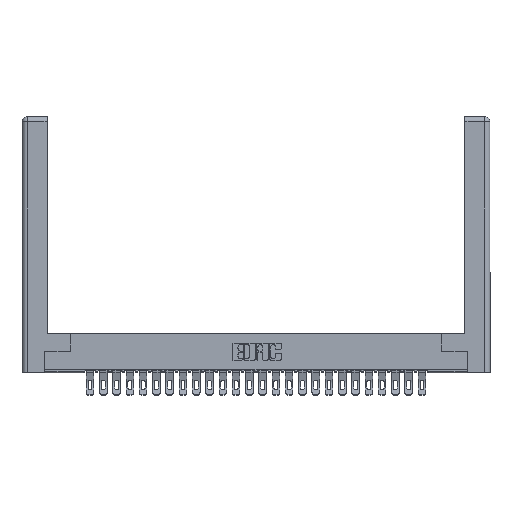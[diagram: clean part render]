
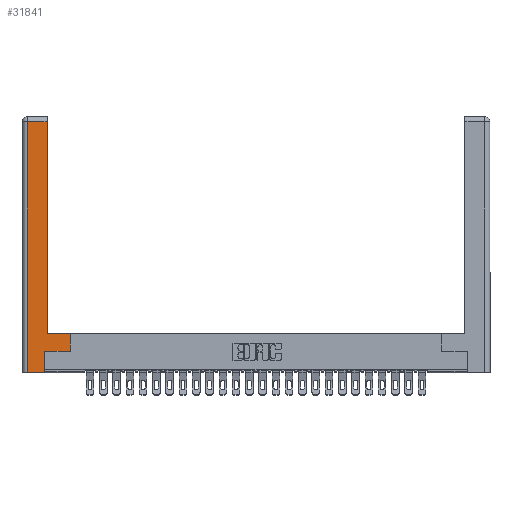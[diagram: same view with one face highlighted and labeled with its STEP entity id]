
A CAD part, top view. The second image highlights one B-rep face of the part: STEP entity #31841.
In plain terms, the highlighted planar face has unit normal (0, 0, 1).
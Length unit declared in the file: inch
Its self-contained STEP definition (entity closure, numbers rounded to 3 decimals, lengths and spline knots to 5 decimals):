
#507 = VECTOR ( 'NONE', #19757, 39.37008 ) ;
#804 = CARTESIAN_POINT ( 'NONE',  ( 0., 0., 0. ) ) ;
#816 = LINE ( 'NONE', #14092, #14166 ) ;
#924 = PLANE ( 'NONE',  #25599 ) ;
#1726 = DIRECTION ( 'NONE',  ( -1., 0., 0. ) ) ;
#2215 = EDGE_CURVE ( 'NONE', #4605, #16464, #33294, .T. ) ;
#2953 = DIRECTION ( 'NONE',  ( 0., -1., 0. ) ) ;
#4559 = CARTESIAN_POINT ( 'NONE',  ( 0.265, 0.245, 0. ) ) ;
#4605 = VERTEX_POINT ( 'NONE', #8911 ) ;
#6234 = DIRECTION ( 'NONE',  ( 0., 0., -1. ) ) ;
#7751 = EDGE_CURVE ( 'NONE', #28301, #33286, #33131, .T. ) ;
#8047 = ORIENTED_EDGE ( 'NONE', *, *, #7751, .T. ) ;
#8273 = CARTESIAN_POINT ( 'NONE',  ( 0.295, 0.45, 0. ) ) ;
#8498 = DIRECTION ( 'NONE',  ( -1., 0., 0. ) ) ;
#8632 = EDGE_CURVE ( 'NONE', #15963, #28950, #816, .T. ) ;
#8840 = ORIENTED_EDGE ( 'NONE', *, *, #24499, .T. ) ;
#8911 = CARTESIAN_POINT ( 'NONE',  ( 0.0615, 0., 0. ) ) ;
#9130 = VECTOR ( 'NONE', #2953, 39.37008 ) ;
#10199 = ORIENTED_EDGE ( 'NONE', *, *, #15983, .T. ) ;
#11151 = VERTEX_POINT ( 'NONE', #18816 ) ;
#12319 = VERTEX_POINT ( 'NONE', #8273 ) ;
#12617 = LINE ( 'NONE', #28324, #30306 ) ;
#12650 = CARTESIAN_POINT ( 'NONE',  ( 0.295, 0.45, 0. ) ) ;
#13372 = DIRECTION ( 'NONE',  ( 0., 1., 0. ) ) ;
#14092 = CARTESIAN_POINT ( 'NONE',  ( 0.565, 0.245, 0. ) ) ;
#14166 = VECTOR ( 'NONE', #32068, 39.37008 ) ;
#14586 = VECTOR ( 'NONE', #8498, 39.37008 ) ;
#14604 = DIRECTION ( 'NONE',  ( 0., 1., 0. ) ) ;
#14971 = EDGE_CURVE ( 'NONE', #12319, #28301, #12617, .T. ) ;
#15002 = DIRECTION ( 'NONE',  ( 1., 0., 0. ) ) ;
#15470 = VECTOR ( 'NONE', #14604, 39.37008 ) ;
#15763 = CARTESIAN_POINT ( 'NONE',  ( 0.565, 0.45, 0. ) ) ;
#15963 = VERTEX_POINT ( 'NONE', #17545 ) ;
#15983 = EDGE_CURVE ( 'NONE', #11151, #12319, #19451, .T. ) ;
#16464 = VERTEX_POINT ( 'NONE', #29003 ) ;
#17545 = CARTESIAN_POINT ( 'NONE',  ( 0.265, 0.245, 0. ) ) ;
#18080 = ORIENTED_EDGE ( 'NONE', *, *, #22861, .T. ) ;
#18816 = CARTESIAN_POINT ( 'NONE',  ( 0.565, 0.45, 0. ) ) ;
#18817 = ORIENTED_EDGE ( 'NONE', *, *, #14971, .T. ) ;
#19451 = LINE ( 'NONE', #12650, #14586 ) ;
#19454 = EDGE_CURVE ( 'NONE', #28950, #11151, #21372, .T. ) ;
#19748 = CARTESIAN_POINT ( 'NONE',  ( 0.295, 2.94, 0. ) ) ;
#19757 = DIRECTION ( 'NONE',  ( -1., 0., 0. ) ) ;
#20015 = ORIENTED_EDGE ( 'NONE', *, *, #2215, .T. ) ;
#21180 = LINE ( 'NONE', #31101, #9130 ) ;
#21372 = LINE ( 'NONE', #15763, #28208 ) ;
#22861 = EDGE_CURVE ( 'NONE', #33286, #4605, #21180, .T. ) ;
#23636 = CARTESIAN_POINT ( 'NONE',  ( 0.565, 0.245, 0. ) ) ;
#24499 = EDGE_CURVE ( 'NONE', #16464, #15963, #30748, .T. ) ;
#24823 = CARTESIAN_POINT ( 'NONE',  ( 0.0615, 2.94, 0. ) ) ;
#25112 = CARTESIAN_POINT ( 'NONE',  ( 0.265, 0., 0. ) ) ;
#25599 = AXIS2_PLACEMENT_3D ( 'NONE', #804, #6234, #1726 ) ;
#26274 = FACE_OUTER_BOUND ( 'NONE', #33277, .T. ) ;
#26662 = ORIENTED_EDGE ( 'NONE', *, *, #19454, .T. ) ;
#26741 = ORIENTED_EDGE ( 'NONE', *, *, #8632, .T. ) ;
#28208 = VECTOR ( 'NONE', #13372, 39.37008 ) ;
#28301 = VERTEX_POINT ( 'NONE', #19748 ) ;
#28324 = CARTESIAN_POINT ( 'NONE',  ( 0.295, 3., 0. ) ) ;
#28950 = VERTEX_POINT ( 'NONE', #23636 ) ;
#29003 = CARTESIAN_POINT ( 'NONE',  ( 0.265, 0., 0. ) ) ;
#29041 = CARTESIAN_POINT ( 'NONE',  ( 0.0615, 2.94, 0. ) ) ;
#30306 = VECTOR ( 'NONE', #33117, 39.37008 ) ;
#30748 = LINE ( 'NONE', #4559, #15470 ) ;
#30873 = VECTOR ( 'NONE', #15002, 39.37008 ) ;
#31101 = CARTESIAN_POINT ( 'NONE',  ( 0.0615, 0., 0. ) ) ;
#31841 = ADVANCED_FACE ( 'NONE', ( #26274 ), #924, .F. ) ;
#32068 = DIRECTION ( 'NONE',  ( 1., 0., 0. ) ) ;
#33117 = DIRECTION ( 'NONE',  ( 0., 1., 0. ) ) ;
#33131 = LINE ( 'NONE', #24823, #507 ) ;
#33277 = EDGE_LOOP ( 'NONE', ( #18817, #8047, #18080, #20015, #8840, #26741, #26662, #10199 ) ) ;
#33286 = VERTEX_POINT ( 'NONE', #29041 ) ;
#33294 = LINE ( 'NONE', #25112, #30873 ) ;
